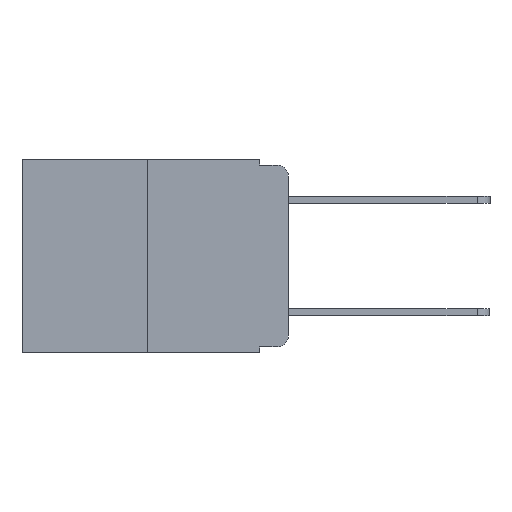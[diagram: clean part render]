
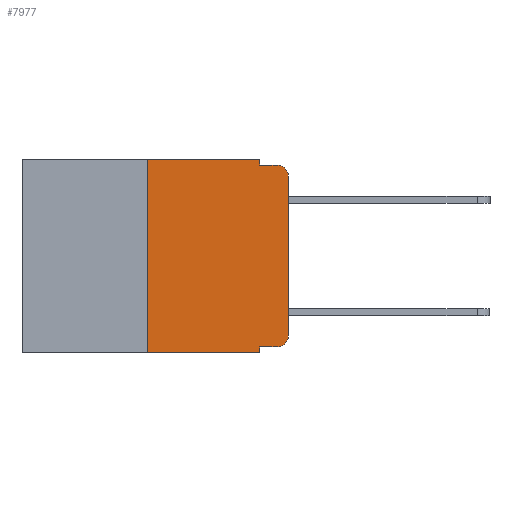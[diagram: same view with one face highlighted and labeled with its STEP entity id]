
A CAD part, left-side view. The second image highlights one B-rep face of the part: STEP entity #7977.
In plain terms, the highlighted planar face has unit normal (-1, 0, 0).
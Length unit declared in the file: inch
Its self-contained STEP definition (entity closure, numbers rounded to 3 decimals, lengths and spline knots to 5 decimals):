
#127 = CARTESIAN_POINT ( 'NONE',  ( 0., 0.473, 0. ) ) ;
#228 = CIRCLE ( 'NONE', #15445, 0.02 ) ;
#241 = CARTESIAN_POINT ( 'NONE',  ( 0., 0.051, -0.01 ) ) ;
#504 = LINE ( 'NONE', #9907, #3631 ) ;
#603 = DIRECTION ( 'NONE',  ( 0., 0., -1. ) ) ;
#767 = ORIENTED_EDGE ( 'NONE', *, *, #7672, .F. ) ;
#1277 = EDGE_CURVE ( 'NONE', #10622, #11326, #504, .T. ) ;
#1336 = CARTESIAN_POINT ( 'NONE',  ( 0., 0., -0.03 ) ) ;
#1397 = FACE_OUTER_BOUND ( 'NONE', #7929, .T. ) ;
#1618 = DIRECTION ( 'NONE',  ( 0., 0., -1. ) ) ;
#1815 = VECTOR ( 'NONE', #3475, 39.37008 ) ;
#1895 = EDGE_CURVE ( 'NONE', #2045, #3379, #8910, .T. ) ;
#2045 = VERTEX_POINT ( 'NONE', #8896 ) ;
#2054 = VERTEX_POINT ( 'NONE', #12983 ) ;
#2108 = ORIENTED_EDGE ( 'NONE', *, *, #1895, .F. ) ;
#2299 = VERTEX_POINT ( 'NONE', #1336 ) ;
#2412 = VERTEX_POINT ( 'NONE', #4255 ) ;
#2539 = EDGE_CURVE ( 'NONE', #10622, #2045, #11468, .T. ) ;
#2624 = ORIENTED_EDGE ( 'NONE', *, *, #6377, .T. ) ;
#2655 = EDGE_CURVE ( 'NONE', #3379, #11993, #12622, .T. ) ;
#3110 = ORIENTED_EDGE ( 'NONE', *, *, #2539, .F. ) ;
#3379 = VERTEX_POINT ( 'NONE', #8902 ) ;
#3475 = DIRECTION ( 'NONE',  ( 0., 0., 1. ) ) ;
#3509 = CARTESIAN_POINT ( 'NONE',  ( 0., 0.25, 0. ) ) ;
#3631 = VECTOR ( 'NONE', #6416, 39.37008 ) ;
#3677 = DIRECTION ( 'NONE',  ( 0., 0., 1. ) ) ;
#4039 = LINE ( 'NONE', #14738, #12681 ) ;
#4255 = CARTESIAN_POINT ( 'NONE',  ( 0., 0.02, -0.333 ) ) ;
#5138 = VECTOR ( 'NONE', #3677, 39.37008 ) ;
#5153 = AXIS2_PLACEMENT_3D ( 'NONE', #127, #9169, #1618 ) ;
#5710 = CARTESIAN_POINT ( 'NONE',  ( 0., 0., 0. ) ) ;
#5953 = EDGE_CURVE ( 'NONE', #2299, #14775, #228, .T. ) ;
#5976 = DIRECTION ( 'NONE',  ( -1., 0., 0. ) ) ;
#6002 = EDGE_CURVE ( 'NONE', #11993, #14775, #11810, .T. ) ;
#6028 = EDGE_CURVE ( 'NONE', #2054, #2299, #8483, .T. ) ;
#6323 = EDGE_CURVE ( 'NONE', #12833, #2412, #11737, .T. ) ;
#6377 = EDGE_CURVE ( 'NONE', #2412, #2054, #10748, .T. ) ;
#6399 = CARTESIAN_POINT ( 'NONE',  ( 0., 0.02, -0.01 ) ) ;
#6416 = DIRECTION ( 'NONE',  ( 0., -1., 0. ) ) ;
#6828 = CARTESIAN_POINT ( 'NONE',  ( 0., 0.02, -0.03 ) ) ;
#6918 = DIRECTION ( 'NONE',  ( 0., -1., 0. ) ) ;
#7351 = ORIENTED_EDGE ( 'NONE', *, *, #6028, .T. ) ;
#7586 = DIRECTION ( 'NONE',  ( 0., -1., 0. ) ) ;
#7672 = EDGE_CURVE ( 'NONE', #12833, #11326, #4039, .T. ) ;
#7741 = ORIENTED_EDGE ( 'NONE', *, *, #6323, .T. ) ;
#7745 = PLANE ( 'NONE',  #5153 ) ;
#7881 = ORIENTED_EDGE ( 'NONE', *, *, #6002, .F. ) ;
#7929 = EDGE_LOOP ( 'NONE', ( #7351, #8314, #7881, #8529, #2108, #3110, #9714, #767, #7741, #2624 ) ) ;
#7959 = CARTESIAN_POINT ( 'NONE',  ( 0., 0.25, -0.343 ) ) ;
#7977 = ADVANCED_FACE ( 'NONE', ( #1397 ), #7745, .F. ) ;
#8165 = CARTESIAN_POINT ( 'NONE',  ( 0., 0.051, -0.333 ) ) ;
#8314 = ORIENTED_EDGE ( 'NONE', *, *, #5953, .T. ) ;
#8339 = DIRECTION ( 'NONE',  ( -1., 0., 0. ) ) ;
#8467 = VECTOR ( 'NONE', #6918, 39.37008 ) ;
#8483 = LINE ( 'NONE', #5710, #5138 ) ;
#8529 = ORIENTED_EDGE ( 'NONE', *, *, #2655, .F. ) ;
#8896 = CARTESIAN_POINT ( 'NONE',  ( 0., 0.25, 0. ) ) ;
#8902 = CARTESIAN_POINT ( 'NONE',  ( 0., 0.051, 0. ) ) ;
#8910 = LINE ( 'NONE', #14171, #14260 ) ;
#8929 = DIRECTION ( 'NONE',  ( 0., -1., 0. ) ) ;
#8934 = VECTOR ( 'NONE', #8929, 39.37008 ) ;
#9169 = DIRECTION ( 'NONE',  ( 1., 0., 0. ) ) ;
#9411 = DIRECTION ( 'NONE',  ( 0., 0., -1. ) ) ;
#9424 = VECTOR ( 'NONE', #13394, 39.37008 ) ;
#9714 = ORIENTED_EDGE ( 'NONE', *, *, #1277, .T. ) ;
#9907 = CARTESIAN_POINT ( 'NONE',  ( 0., 0.473, -0.343 ) ) ;
#9999 = CARTESIAN_POINT ( 'NONE',  ( 0., 0.051, 0. ) ) ;
#10061 = CARTESIAN_POINT ( 'NONE',  ( 0., 0.051, -0.01 ) ) ;
#10622 = VERTEX_POINT ( 'NONE', #7959 ) ;
#10748 = CIRCLE ( 'NONE', #10837, 0.02 ) ;
#10837 = AXIS2_PLACEMENT_3D ( 'NONE', #14800, #8339, #603 ) ;
#10934 = CARTESIAN_POINT ( 'NONE',  ( 0., 0.051, -0.343 ) ) ;
#11326 = VERTEX_POINT ( 'NONE', #10934 ) ;
#11468 = LINE ( 'NONE', #3509, #1815 ) ;
#11737 = LINE ( 'NONE', #8165, #8467 ) ;
#11810 = LINE ( 'NONE', #10061, #8934 ) ;
#11993 = VERTEX_POINT ( 'NONE', #241 ) ;
#12622 = LINE ( 'NONE', #9999, #9424 ) ;
#12681 = VECTOR ( 'NONE', #9411, 39.37008 ) ;
#12833 = VERTEX_POINT ( 'NONE', #14109 ) ;
#12983 = CARTESIAN_POINT ( 'NONE',  ( 0., 0., -0.313 ) ) ;
#13394 = DIRECTION ( 'NONE',  ( 0., 0., -1. ) ) ;
#13926 = DIRECTION ( 'NONE',  ( 0., 0., -1. ) ) ;
#14109 = CARTESIAN_POINT ( 'NONE',  ( 0., 0.051, -0.333 ) ) ;
#14171 = CARTESIAN_POINT ( 'NONE',  ( 0., 0.473, 0. ) ) ;
#14260 = VECTOR ( 'NONE', #7586, 39.37008 ) ;
#14738 = CARTESIAN_POINT ( 'NONE',  ( 0., 0.051, 0. ) ) ;
#14775 = VERTEX_POINT ( 'NONE', #6399 ) ;
#14800 = CARTESIAN_POINT ( 'NONE',  ( 0., 0.02, -0.313 ) ) ;
#15445 = AXIS2_PLACEMENT_3D ( 'NONE', #6828, #5976, #13926 ) ;
